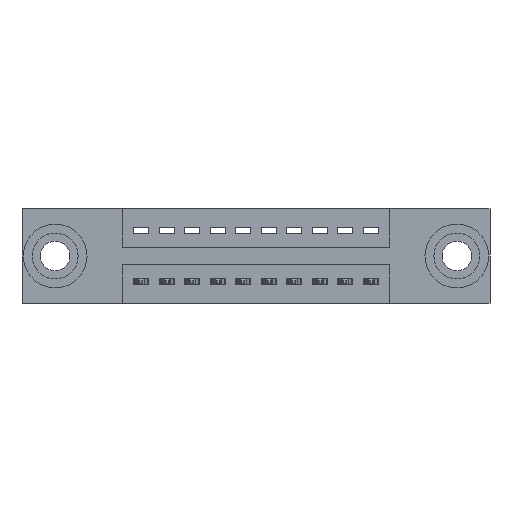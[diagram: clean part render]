
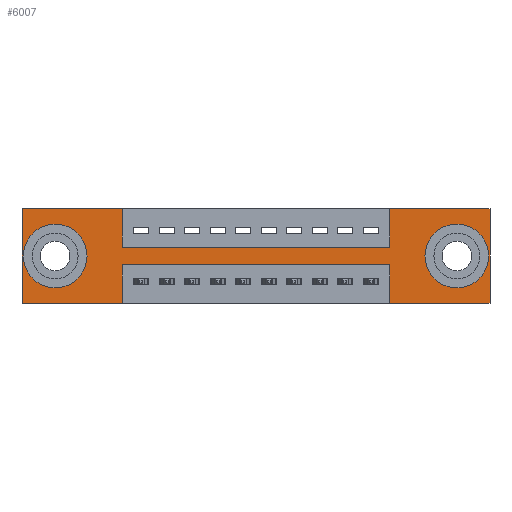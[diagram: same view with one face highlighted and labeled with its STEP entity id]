
A CAD part, front view. The second image highlights one B-rep face of the part: STEP entity #6007.
In plain terms, the highlighted planar face has unit normal (0, -1, 0).
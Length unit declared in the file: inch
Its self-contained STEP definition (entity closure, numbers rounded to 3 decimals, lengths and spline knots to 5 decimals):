
#84 = VECTOR ( 'NONE', #4063, 39.37008 ) ;
#310 = EDGE_CURVE ( 'NONE', #7581, #2464, #3478, .T. ) ;
#507 = CARTESIAN_POINT ( 'NONE',  ( 0., 0., 0. ) ) ;
#548 = LINE ( 'NONE', #3499, #8166 ) ;
#554 = CARTESIAN_POINT ( 'NONE',  ( 1.705, 0., -0.107 ) ) ;
#601 = ORIENTED_EDGE ( 'NONE', *, *, #7762, .F. ) ;
#710 = CARTESIAN_POINT ( 'NONE',  ( 1.705, 0., -0.263 ) ) ;
#910 = VERTEX_POINT ( 'NONE', #8683 ) ;
#929 = EDGE_CURVE ( 'NONE', #10888, #4522, #8395, .T. ) ;
#1159 = CARTESIAN_POINT ( 'NONE',  ( 0.3925, 0., -0.37 ) ) ;
#1235 = CARTESIAN_POINT ( 'NONE',  ( 0.3925, 0., 0. ) ) ;
#1296 = CARTESIAN_POINT ( 'NONE',  ( 0.3925, 0., 0. ) ) ;
#1316 = EDGE_CURVE ( 'NONE', #7478, #9660, #4587, .T. ) ;
#1409 = EDGE_CURVE ( 'NONE', #7127, #12512, #11609, .T. ) ;
#1441 = CARTESIAN_POINT ( 'NONE',  ( 0.13, 0., -0.185 ) ) ;
#1467 = CARTESIAN_POINT ( 'NONE',  ( 1.835, 0., -0.37 ) ) ;
#1671 = CARTESIAN_POINT ( 'NONE',  ( 0., 0., 0. ) ) ;
#1718 = ORIENTED_EDGE ( 'NONE', *, *, #1316, .T. ) ;
#1723 = VECTOR ( 'NONE', #8972, 39.37008 ) ;
#1813 = LINE ( 'NONE', #9541, #6746 ) ;
#1855 = EDGE_LOOP ( 'NONE', ( #5844, #5392 ) ) ;
#1926 = CARTESIAN_POINT ( 'NONE',  ( 1.4425, 0., 0. ) ) ;
#2297 = CARTESIAN_POINT ( 'NONE',  ( 1.4425, 0., -0.37 ) ) ;
#2464 = VERTEX_POINT ( 'NONE', #1467 ) ;
#2508 = DIRECTION ( 'NONE',  ( 0., 0., 1. ) ) ;
#2690 = CARTESIAN_POINT ( 'NONE',  ( 1.4425, 0., -0.15 ) ) ;
#2703 = LINE ( 'NONE', #10820, #9701 ) ;
#2787 = EDGE_LOOP ( 'NONE', ( #4331, #1718 ) ) ;
#3255 = CIRCLE ( 'NONE', #11460, 0.078 ) ;
#3290 = VECTOR ( 'NONE', #3812, 39.37008 ) ;
#3292 = VECTOR ( 'NONE', #5679, 39.37008 ) ;
#3386 = CARTESIAN_POINT ( 'NONE',  ( 1.835, 0., 0. ) ) ;
#3417 = VERTEX_POINT ( 'NONE', #12450 ) ;
#3478 = LINE ( 'NONE', #3386, #8263 ) ;
#3482 = CARTESIAN_POINT ( 'NONE',  ( 1.4425, 0., -0.37 ) ) ;
#3492 = EDGE_CURVE ( 'NONE', #8941, #9668, #3255, .T. ) ;
#3499 = CARTESIAN_POINT ( 'NONE',  ( 0., 0., 0. ) ) ;
#3598 = DIRECTION ( 'NONE',  ( 1., 0., 0. ) ) ;
#3677 = CARTESIAN_POINT ( 'NONE',  ( 0.3925, 0., -0.15 ) ) ;
#3812 = DIRECTION ( 'NONE',  ( 0., 0., 1. ) ) ;
#3906 = VECTOR ( 'NONE', #4011, 39.37008 ) ;
#4011 = DIRECTION ( 'NONE',  ( 0., 0., 1. ) ) ;
#4063 = DIRECTION ( 'NONE',  ( 0., 0., -1. ) ) ;
#4216 = FACE_OUTER_BOUND ( 'NONE', #6462, .T. ) ;
#4331 = ORIENTED_EDGE ( 'NONE', *, *, #5615, .T. ) ;
#4423 = VERTEX_POINT ( 'NONE', #4548 ) ;
#4522 = VERTEX_POINT ( 'NONE', #3677 ) ;
#4548 = CARTESIAN_POINT ( 'NONE',  ( 1.4425, 0., 0. ) ) ;
#4553 = EDGE_CURVE ( 'NONE', #4423, #7581, #548, .T. ) ;
#4573 = DIRECTION ( 'NONE',  ( 0., 0., -1. ) ) ;
#4584 = CARTESIAN_POINT ( 'NONE',  ( 1.705, 0., -0.185 ) ) ;
#4587 = CIRCLE ( 'NONE', #6170, 0.078 ) ;
#4629 = CARTESIAN_POINT ( 'NONE',  ( 0., 0., 0. ) ) ;
#4643 = DIRECTION ( 'NONE',  ( 0., 1., 0. ) ) ;
#4651 = CARTESIAN_POINT ( 'NONE',  ( 1.705, 0., -0.185 ) ) ;
#4703 = DIRECTION ( 'NONE',  ( 0., 1., 0. ) ) ;
#5053 = CARTESIAN_POINT ( 'NONE',  ( 1.835, 0., 0. ) ) ;
#5242 = DIRECTION ( 'NONE',  ( -1., 0., 0. ) ) ;
#5392 = ORIENTED_EDGE ( 'NONE', *, *, #3492, .T. ) ;
#5401 = VERTEX_POINT ( 'NONE', #12263 ) ;
#5473 = ORIENTED_EDGE ( 'NONE', *, *, #10347, .F. ) ;
#5521 = DIRECTION ( 'NONE',  ( 0., 0., -1. ) ) ;
#5615 = EDGE_CURVE ( 'NONE', #9660, #7478, #8339, .T. ) ;
#5679 = DIRECTION ( 'NONE',  ( 0., 0., 1. ) ) ;
#5689 = ORIENTED_EDGE ( 'NONE', *, *, #929, .F. ) ;
#5797 = CARTESIAN_POINT ( 'NONE',  ( 1.4425, 0., -0.22 ) ) ;
#5844 = ORIENTED_EDGE ( 'NONE', *, *, #9524, .T. ) ;
#6007 = ADVANCED_FACE ( 'NONE', ( #11565, #6716, #4216 ), #10584, .T. ) ;
#6056 = CIRCLE ( 'NONE', #10983, 0.078 ) ;
#6082 = LINE ( 'NONE', #9809, #12478 ) ;
#6170 = AXIS2_PLACEMENT_3D ( 'NONE', #4584, #4643, #6505 ) ;
#6462 = EDGE_LOOP ( 'NONE', ( #6604, #7831, #7913, #12489, #10611, #11507, #10329, #10898, #5689, #5473, #7253, #601 ) ) ;
#6505 = DIRECTION ( 'NONE',  ( 0., 0., -1. ) ) ;
#6604 = ORIENTED_EDGE ( 'NONE', *, *, #12140, .F. ) ;
#6716 = FACE_BOUND ( 'NONE', #1855, .T. ) ;
#6746 = VECTOR ( 'NONE', #6797, 39.37008 ) ;
#6797 = DIRECTION ( 'NONE',  ( -1., 0., 0. ) ) ;
#6991 = CARTESIAN_POINT ( 'NONE',  ( 0.3925, 0., -0.15 ) ) ;
#7127 = VERTEX_POINT ( 'NONE', #2297 ) ;
#7253 = ORIENTED_EDGE ( 'NONE', *, *, #10419, .F. ) ;
#7281 = CARTESIAN_POINT ( 'NONE',  ( 0.13, 0., -0.263 ) ) ;
#7478 = VERTEX_POINT ( 'NONE', #710 ) ;
#7553 = LINE ( 'NONE', #1159, #1723 ) ;
#7581 = VERTEX_POINT ( 'NONE', #5053 ) ;
#7606 = AXIS2_PLACEMENT_3D ( 'NONE', #4651, #4703, #4573 ) ;
#7762 = EDGE_CURVE ( 'NONE', #5401, #910, #2703, .T. ) ;
#7799 = VECTOR ( 'NONE', #8841, 39.37008 ) ;
#7831 = ORIENTED_EDGE ( 'NONE', *, *, #8752, .F. ) ;
#7913 = ORIENTED_EDGE ( 'NONE', *, *, #1409, .F. ) ;
#8048 = VERTEX_POINT ( 'NONE', #1671 ) ;
#8166 = VECTOR ( 'NONE', #3598, 39.37008 ) ;
#8263 = VECTOR ( 'NONE', #5521, 39.37008 ) ;
#8285 = DIRECTION ( 'NONE',  ( 0., 1., 0. ) ) ;
#8339 = CIRCLE ( 'NONE', #7606, 0.078 ) ;
#8395 = LINE ( 'NONE', #1296, #84 ) ;
#8484 = CARTESIAN_POINT ( 'NONE',  ( 0.13, 0., -0.107 ) ) ;
#8665 = LINE ( 'NONE', #507, #3292 ) ;
#8683 = CARTESIAN_POINT ( 'NONE',  ( 0., 0., -0.37 ) ) ;
#8752 = EDGE_CURVE ( 'NONE', #12512, #3417, #6082, .T. ) ;
#8841 = DIRECTION ( 'NONE',  ( 1., 0., 0. ) ) ;
#8941 = VERTEX_POINT ( 'NONE', #7281 ) ;
#8972 = DIRECTION ( 'NONE',  ( 0., 0., -1. ) ) ;
#9103 = VERTEX_POINT ( 'NONE', #2690 ) ;
#9240 = LINE ( 'NONE', #4629, #11612 ) ;
#9524 = EDGE_CURVE ( 'NONE', #9668, #8941, #6056, .T. ) ;
#9541 = CARTESIAN_POINT ( 'NONE',  ( 0., 0., -0.37 ) ) ;
#9660 = VERTEX_POINT ( 'NONE', #554 ) ;
#9668 = VERTEX_POINT ( 'NONE', #8484 ) ;
#9701 = VECTOR ( 'NONE', #10775, 39.37008 ) ;
#9809 = CARTESIAN_POINT ( 'NONE',  ( 0.3925, 0., -0.22 ) ) ;
#10043 = EDGE_CURVE ( 'NONE', #4522, #9103, #12320, .T. ) ;
#10329 = ORIENTED_EDGE ( 'NONE', *, *, #11240, .F. ) ;
#10347 = EDGE_CURVE ( 'NONE', #8048, #10888, #9240, .T. ) ;
#10419 = EDGE_CURVE ( 'NONE', #910, #8048, #8665, .T. ) ;
#10498 = DIRECTION ( 'NONE',  ( 0., 0., -1. ) ) ;
#10536 = DIRECTION ( 'NONE',  ( 0., -1., 0. ) ) ;
#10553 = CARTESIAN_POINT ( 'NONE',  ( 0., 0., -0.37 ) ) ;
#10584 = PLANE ( 'NONE',  #11030 ) ;
#10611 = ORIENTED_EDGE ( 'NONE', *, *, #310, .F. ) ;
#10775 = DIRECTION ( 'NONE',  ( -1., 0., 0. ) ) ;
#10820 = CARTESIAN_POINT ( 'NONE',  ( 0., 0., -0.37 ) ) ;
#10888 = VERTEX_POINT ( 'NONE', #1235 ) ;
#10898 = ORIENTED_EDGE ( 'NONE', *, *, #10043, .F. ) ;
#10983 = AXIS2_PLACEMENT_3D ( 'NONE', #1441, #8285, #2508 ) ;
#11026 = LINE ( 'NONE', #1926, #3906 ) ;
#11030 = AXIS2_PLACEMENT_3D ( 'NONE', #10553, #10536, #10498 ) ;
#11040 = DIRECTION ( 'NONE',  ( 1., 0., 0. ) ) ;
#11185 = EDGE_CURVE ( 'NONE', #2464, #7127, #1813, .T. ) ;
#11240 = EDGE_CURVE ( 'NONE', #9103, #4423, #11026, .T. ) ;
#11460 = AXIS2_PLACEMENT_3D ( 'NONE', #11911, #11894, #11858 ) ;
#11507 = ORIENTED_EDGE ( 'NONE', *, *, #4553, .F. ) ;
#11565 = FACE_BOUND ( 'NONE', #2787, .T. ) ;
#11609 = LINE ( 'NONE', #3482, #3290 ) ;
#11612 = VECTOR ( 'NONE', #11040, 39.37008 ) ;
#11858 = DIRECTION ( 'NONE',  ( 0., 0., 1. ) ) ;
#11894 = DIRECTION ( 'NONE',  ( 0., 1., 0. ) ) ;
#11911 = CARTESIAN_POINT ( 'NONE',  ( 0.13, 0., -0.185 ) ) ;
#12140 = EDGE_CURVE ( 'NONE', #3417, #5401, #7553, .T. ) ;
#12263 = CARTESIAN_POINT ( 'NONE',  ( 0.3925, 0., -0.37 ) ) ;
#12320 = LINE ( 'NONE', #6991, #7799 ) ;
#12450 = CARTESIAN_POINT ( 'NONE',  ( 0.3925, 0., -0.22 ) ) ;
#12478 = VECTOR ( 'NONE', #5242, 39.37008 ) ;
#12489 = ORIENTED_EDGE ( 'NONE', *, *, #11185, .F. ) ;
#12512 = VERTEX_POINT ( 'NONE', #5797 ) ;
